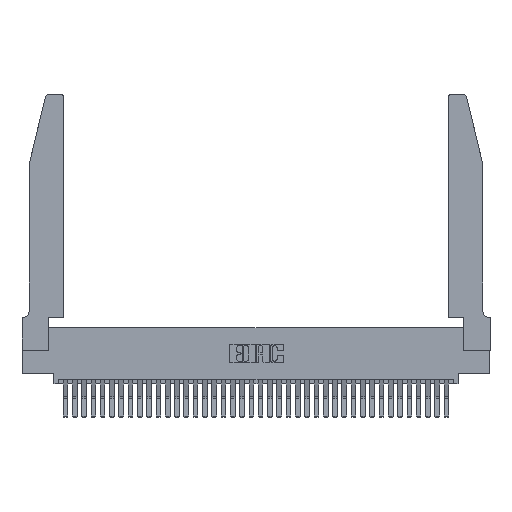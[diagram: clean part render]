
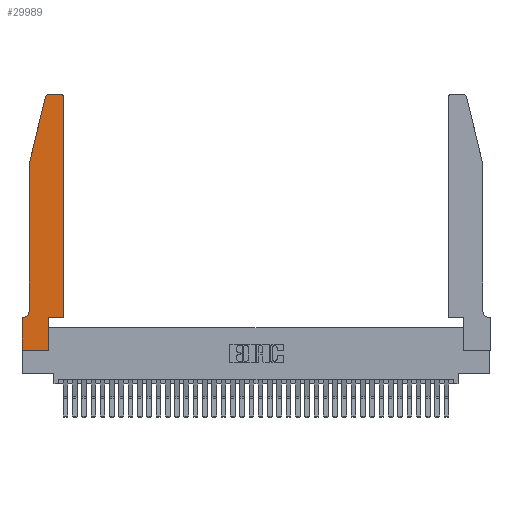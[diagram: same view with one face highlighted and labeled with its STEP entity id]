
A CAD part, top view. The second image highlights one B-rep face of the part: STEP entity #29989.
In plain terms, the highlighted planar face has unit normal (0, 0, 1).
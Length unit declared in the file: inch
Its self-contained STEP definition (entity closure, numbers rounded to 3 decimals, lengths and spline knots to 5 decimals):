
#121 = CARTESIAN_POINT ( 'NONE',  ( 0.4505, 0.35, 0.37 ) ) ;
#213 = VECTOR ( 'NONE', #24101, 39.37008 ) ;
#801 = VERTEX_POINT ( 'NONE', #21116 ) ;
#831 = LINE ( 'NONE', #36713, #7785 ) ;
#1085 = AXIS2_PLACEMENT_3D ( 'NONE', #17694, #20637, #2953 ) ;
#1625 = VERTEX_POINT ( 'NONE', #20224 ) ;
#1846 = CARTESIAN_POINT ( 'NONE',  ( 0.2605, 2.75, 0.37 ) ) ;
#2068 = EDGE_CURVE ( 'NONE', #28512, #801, #24967, .T. ) ;
#2287 = VECTOR ( 'NONE', #22227, 39.37008 ) ;
#2621 = VERTEX_POINT ( 'NONE', #32893 ) ;
#2925 = CARTESIAN_POINT ( 'NONE',  ( 0.4205, 2.75, 0.37 ) ) ;
#2953 = DIRECTION ( 'NONE',  ( 1., 0., 0. ) ) ;
#3144 = VERTEX_POINT ( 'NONE', #35398 ) ;
#3837 = LINE ( 'NONE', #11612, #10710 ) ;
#3870 = EDGE_CURVE ( 'NONE', #8622, #12287, #16035, .T. ) ;
#5198 = ORIENTED_EDGE ( 'NONE', *, *, #6489, .T. ) ;
#6001 = CARTESIAN_POINT ( 'NONE',  ( 0., 0., 0.37 ) ) ;
#6280 = VERTEX_POINT ( 'NONE', #6001 ) ;
#6489 = EDGE_CURVE ( 'NONE', #801, #29941, #30408, .T. ) ;
#6806 = EDGE_CURVE ( 'NONE', #12287, #28512, #3837, .T. ) ;
#7785 = VECTOR ( 'NONE', #19389, 39.37008 ) ;
#7801 = VECTOR ( 'NONE', #23011, 39.37008 ) ;
#8622 = VERTEX_POINT ( 'NONE', #16141 ) ;
#8940 = VECTOR ( 'NONE', #28409, 39.37008 ) ;
#9086 = ORIENTED_EDGE ( 'NONE', *, *, #32194, .T. ) ;
#9408 = CARTESIAN_POINT ( 'NONE',  ( 0.4205, 2.72, 0.37 ) ) ;
#9617 = LINE ( 'NONE', #20098, #7801 ) ;
#9912 = CARTESIAN_POINT ( 'NONE',  ( 0.0755, 0.35, 0.37 ) ) ;
#10184 = CARTESIAN_POINT ( 'NONE',  ( 0.0055, 0.42, 0.37 ) ) ;
#10322 = CARTESIAN_POINT ( 'NONE',  ( 0., 0., 0.37 ) ) ;
#10710 = VECTOR ( 'NONE', #14637, 39.37008 ) ;
#11463 = AXIS2_PLACEMENT_3D ( 'NONE', #10184, #30655, #13210 ) ;
#11612 = CARTESIAN_POINT ( 'NONE',  ( 0.0755, 2., 0.37 ) ) ;
#11875 = CARTESIAN_POINT ( 'NONE',  ( 0.284, 2.72, 0.37 ) ) ;
#12287 = VERTEX_POINT ( 'NONE', #20415 ) ;
#12442 = DIRECTION ( 'NONE',  ( 1., 0., 0. ) ) ;
#12527 = CARTESIAN_POINT ( 'NONE',  ( 0.2865, 0.35, 0.37 ) ) ;
#13175 = EDGE_CURVE ( 'NONE', #26797, #1625, #16898, .T. ) ;
#13210 = DIRECTION ( 'NONE',  ( -1., 0., 0. ) ) ;
#13430 = EDGE_LOOP ( 'NONE', ( #13846, #9086, #17543, #30341, #32173, #5198, #19398, #17566, #26137, #18641, #21384, #15862 ) ) ;
#13846 = ORIENTED_EDGE ( 'NONE', *, *, #13175, .T. ) ;
#14592 = CARTESIAN_POINT ( 'NONE',  ( 0., 0.35, 0.37 ) ) ;
#14637 = DIRECTION ( 'NONE',  ( 0., -1., 0. ) ) ;
#14898 = DIRECTION ( 'NONE',  ( 1., 0., 0. ) ) ;
#15530 = DIRECTION ( 'NONE',  ( 0., 1., 0. ) ) ;
#15862 = ORIENTED_EDGE ( 'NONE', *, *, #26944, .T. ) ;
#16035 = LINE ( 'NONE', #21211, #213 ) ;
#16141 = CARTESIAN_POINT ( 'NONE',  ( 0.25487, 2.72718, 0.37 ) ) ;
#16898 = LINE ( 'NONE', #1846, #8940 ) ;
#17121 = LINE ( 'NONE', #10322, #2287 ) ;
#17185 = CARTESIAN_POINT ( 'NONE',  ( 0.4505, 2.72, 0.37 ) ) ;
#17543 = ORIENTED_EDGE ( 'NONE', *, *, #3870, .T. ) ;
#17566 = ORIENTED_EDGE ( 'NONE', *, *, #27164, .T. ) ;
#17594 = CIRCLE ( 'NONE', #35867, 0.03 ) ;
#17694 = CARTESIAN_POINT ( 'NONE',  ( 0., 0.35, 0.37 ) ) ;
#18641 = ORIENTED_EDGE ( 'NONE', *, *, #33743, .T. ) ;
#19321 = CIRCLE ( 'NONE', #28721, 0.03 ) ;
#19389 = DIRECTION ( 'NONE',  ( 0., -1., 0. ) ) ;
#19398 = ORIENTED_EDGE ( 'NONE', *, *, #22880, .T. ) ;
#20098 = CARTESIAN_POINT ( 'NONE',  ( 0.4505, 0.35, 0.37 ) ) ;
#20224 = CARTESIAN_POINT ( 'NONE',  ( 0.284, 2.75, 0.37 ) ) ;
#20415 = CARTESIAN_POINT ( 'NONE',  ( 0.0755, 2., 0.37 ) ) ;
#20637 = DIRECTION ( 'NONE',  ( 0., 0., 1. ) ) ;
#21116 = CARTESIAN_POINT ( 'NONE',  ( 0.0055, 0.35, 0.37 ) ) ;
#21211 = CARTESIAN_POINT ( 'NONE',  ( 0.0755, 2., 0.37 ) ) ;
#21384 = ORIENTED_EDGE ( 'NONE', *, *, #30410, .T. ) ;
#22227 = DIRECTION ( 'NONE',  ( 1., 0., 0. ) ) ;
#22624 = FACE_OUTER_BOUND ( 'NONE', #13430, .T. ) ;
#22654 = EDGE_CURVE ( 'NONE', #2621, #3144, #30698, .T. ) ;
#22880 = EDGE_CURVE ( 'NONE', #29941, #6280, #831, .T. ) ;
#23011 = DIRECTION ( 'NONE',  ( 0., 1., 0. ) ) ;
#24101 = DIRECTION ( 'NONE',  ( -0.239, -0.971, 0. ) ) ;
#24967 = CIRCLE ( 'NONE', #11463, 0.07 ) ;
#25527 = VECTOR ( 'NONE', #33824, 39.37008 ) ;
#26137 = ORIENTED_EDGE ( 'NONE', *, *, #22654, .T. ) ;
#26309 = PLANE ( 'NONE',  #1085 ) ;
#26797 = VERTEX_POINT ( 'NONE', #2925 ) ;
#26944 = EDGE_CURVE ( 'NONE', #35908, #26797, #17594, .T. ) ;
#27164 = EDGE_CURVE ( 'NONE', #6280, #2621, #17121, .T. ) ;
#28409 = DIRECTION ( 'NONE',  ( -1., 0., 0. ) ) ;
#28512 = VERTEX_POINT ( 'NONE', #28671 ) ;
#28671 = CARTESIAN_POINT ( 'NONE',  ( 0.0755, 0.42, 0.37 ) ) ;
#28721 = AXIS2_PLACEMENT_3D ( 'NONE', #11875, #32274, #14898 ) ;
#29783 = VECTOR ( 'NONE', #15530, 39.37008 ) ;
#29913 = DIRECTION ( 'NONE',  ( 0., 0., 1. ) ) ;
#29941 = VERTEX_POINT ( 'NONE', #14592 ) ;
#29989 = ADVANCED_FACE ( 'NONE', ( #22624 ), #26309, .T. ) ;
#30341 = ORIENTED_EDGE ( 'NONE', *, *, #6806, .T. ) ;
#30408 = LINE ( 'NONE', #9912, #37224 ) ;
#30410 = EDGE_CURVE ( 'NONE', #33394, #35908, #9617, .T. ) ;
#30655 = DIRECTION ( 'NONE',  ( 0., 0., -1. ) ) ;
#30698 = LINE ( 'NONE', #12527, #29783 ) ;
#30795 = CARTESIAN_POINT ( 'NONE',  ( 0.4505, 0.35, 0.37 ) ) ;
#32173 = ORIENTED_EDGE ( 'NONE', *, *, #2068, .T. ) ;
#32194 = EDGE_CURVE ( 'NONE', #1625, #8622, #19321, .T. ) ;
#32274 = DIRECTION ( 'NONE',  ( 0., 0., 1. ) ) ;
#32893 = CARTESIAN_POINT ( 'NONE',  ( 0.2865, 0., 0.37 ) ) ;
#33394 = VERTEX_POINT ( 'NONE', #121 ) ;
#33743 = EDGE_CURVE ( 'NONE', #3144, #33394, #34110, .T. ) ;
#33824 = DIRECTION ( 'NONE',  ( 1., 0., 0. ) ) ;
#34110 = LINE ( 'NONE', #30795, #25527 ) ;
#35398 = CARTESIAN_POINT ( 'NONE',  ( 0.2865, 0.35, 0.37 ) ) ;
#35867 = AXIS2_PLACEMENT_3D ( 'NONE', #9408, #29913, #12442 ) ;
#35908 = VERTEX_POINT ( 'NONE', #17185 ) ;
#36237 = DIRECTION ( 'NONE',  ( -1., 0., 0. ) ) ;
#36713 = CARTESIAN_POINT ( 'NONE',  ( 0., 0., 0.37 ) ) ;
#37224 = VECTOR ( 'NONE', #36237, 39.37008 ) ;
